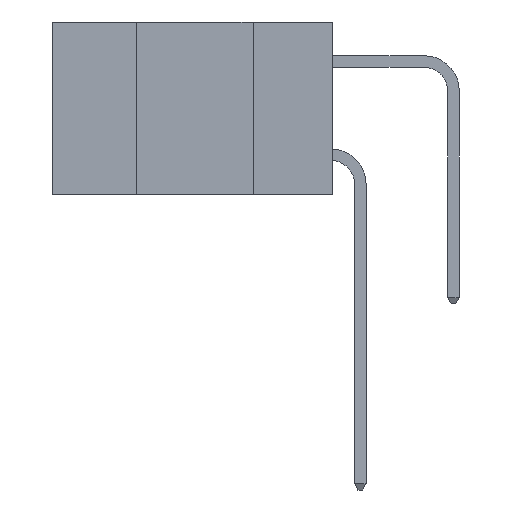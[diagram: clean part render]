
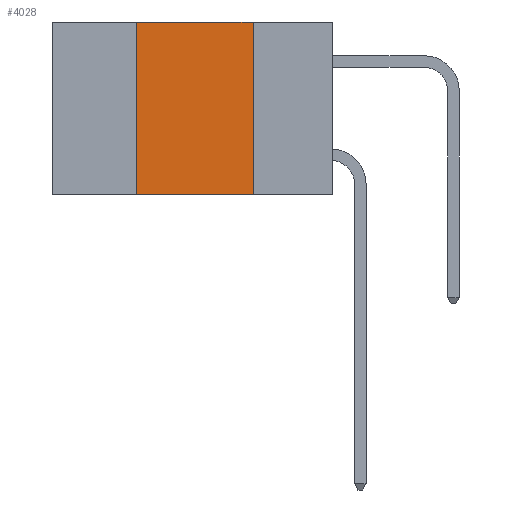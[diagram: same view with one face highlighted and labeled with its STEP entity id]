
A CAD part, left-side view. The second image highlights one B-rep face of the part: STEP entity #4028.
In plain terms, the highlighted planar face has unit normal (-1, 0, 0).
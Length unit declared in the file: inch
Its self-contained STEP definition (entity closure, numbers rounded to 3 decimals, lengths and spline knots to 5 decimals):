
#219 = EDGE_CURVE ( 'NONE', #6288, #4425, #16684, .T. ) ;
#264 = FACE_OUTER_BOUND ( 'NONE', #15627, .T. ) ;
#900 = DIRECTION ( 'NONE',  ( 0., 0., -1. ) ) ;
#1093 = DIRECTION ( 'NONE',  ( 1., 0., 0. ) ) ;
#1129 = VECTOR ( 'NONE', #12574, 39.37008 ) ;
#1165 = CARTESIAN_POINT ( 'NONE',  ( 0., 0.6, 0. ) ) ;
#2153 = PLANE ( 'NONE',  #16553 ) ;
#2446 = VERTEX_POINT ( 'NONE', #12929 ) ;
#2547 = LINE ( 'NONE', #4536, #5339 ) ;
#3124 = EDGE_CURVE ( 'NONE', #17714, #6288, #15295, .T. ) ;
#4028 = ADVANCED_FACE ( 'NONE', ( #264 ), #2153, .F. ) ;
#4241 = ORIENTED_EDGE ( 'NONE', *, *, #219, .F. ) ;
#4425 = VERTEX_POINT ( 'NONE', #10312 ) ;
#4437 = DIRECTION ( 'NONE',  ( 0., -1., 0. ) ) ;
#4470 = CARTESIAN_POINT ( 'NONE',  ( 0., 0.17, 0. ) ) ;
#4536 = CARTESIAN_POINT ( 'NONE',  ( 0., 0.6, -0.37 ) ) ;
#4845 = LINE ( 'NONE', #10006, #1129 ) ;
#5339 = VECTOR ( 'NONE', #4437, 39.37008 ) ;
#5474 = VECTOR ( 'NONE', #10635, 39.37008 ) ;
#5928 = ORIENTED_EDGE ( 'NONE', *, *, #7742, .F. ) ;
#6288 = VERTEX_POINT ( 'NONE', #4470 ) ;
#7742 = EDGE_CURVE ( 'NONE', #2446, #17714, #4845, .T. ) ;
#7847 = CARTESIAN_POINT ( 'NONE',  ( 0., 0.42, 0. ) ) ;
#10006 = CARTESIAN_POINT ( 'NONE',  ( 0., 0.42, -0.37 ) ) ;
#10312 = CARTESIAN_POINT ( 'NONE',  ( 0., 0.17, -0.37 ) ) ;
#10635 = DIRECTION ( 'NONE',  ( 0., 0., -1. ) ) ;
#11565 = VECTOR ( 'NONE', #17085, 39.37008 ) ;
#11577 = EDGE_CURVE ( 'NONE', #2446, #4425, #2547, .T. ) ;
#12574 = DIRECTION ( 'NONE',  ( 0., 0., 1. ) ) ;
#12929 = CARTESIAN_POINT ( 'NONE',  ( 0., 0.42, -0.37 ) ) ;
#13261 = CARTESIAN_POINT ( 'NONE',  ( 0., 0.6, 0. ) ) ;
#14171 = ORIENTED_EDGE ( 'NONE', *, *, #11577, .T. ) ;
#15295 = LINE ( 'NONE', #13261, #11565 ) ;
#15627 = EDGE_LOOP ( 'NONE', ( #4241, #17209, #5928, #14171 ) ) ;
#16553 = AXIS2_PLACEMENT_3D ( 'NONE', #1165, #1093, #900 ) ;
#16651 = CARTESIAN_POINT ( 'NONE',  ( 0., 0.17, -0.37 ) ) ;
#16684 = LINE ( 'NONE', #16651, #5474 ) ;
#17085 = DIRECTION ( 'NONE',  ( 0., -1., 0. ) ) ;
#17209 = ORIENTED_EDGE ( 'NONE', *, *, #3124, .F. ) ;
#17714 = VERTEX_POINT ( 'NONE', #7847 ) ;
